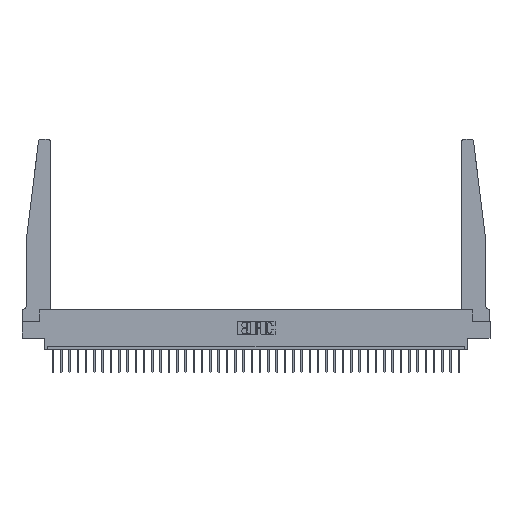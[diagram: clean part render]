
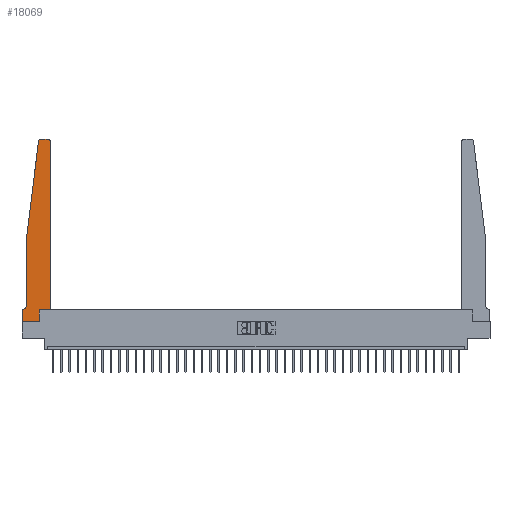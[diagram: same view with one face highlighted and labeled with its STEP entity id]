
A CAD part, top view. The second image highlights one B-rep face of the part: STEP entity #18069.
In plain terms, the highlighted planar face has unit normal (0, 0, 1).
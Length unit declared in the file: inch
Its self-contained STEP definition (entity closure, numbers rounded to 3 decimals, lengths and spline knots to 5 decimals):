
#10 = AXIS2_PLACEMENT_3D ( 'NONE', #720, #8918, #19592 ) ;
#615 = EDGE_CURVE ( 'NONE', #26898, #22682, #21179, .T. ) ;
#720 = CARTESIAN_POINT ( 'NONE',  ( 0.015, 0.2375, 0.37 ) ) ;
#728 = DIRECTION ( 'NONE',  ( 0., 0., 1. ) ) ;
#756 = CARTESIAN_POINT ( 'NONE',  ( 0.065, 1.25, 0.37 ) ) ;
#1066 = EDGE_CURVE ( 'NONE', #21076, #34703, #13447, .T. ) ;
#1390 = CARTESIAN_POINT ( 'NONE',  ( 0.065, 1.25, 0.37 ) ) ;
#3433 = CARTESIAN_POINT ( 'NONE',  ( 0.395, 2.72, 0.37 ) ) ;
#3521 = VECTOR ( 'NONE', #23719, 39.37008 ) ;
#3682 = ORIENTED_EDGE ( 'NONE', *, *, #18280, .T. ) ;
#3773 = LINE ( 'NONE', #25490, #32810 ) ;
#3813 = LINE ( 'NONE', #27204, #4213 ) ;
#3854 = CARTESIAN_POINT ( 'NONE',  ( 0.2605, 0.18, 0.37 ) ) ;
#4213 = VECTOR ( 'NONE', #9031, 39.37008 ) ;
#4278 = VECTOR ( 'NONE', #23794, 39.37008 ) ;
#5318 = FACE_OUTER_BOUND ( 'NONE', #15963, .T. ) ;
#5450 = CARTESIAN_POINT ( 'NONE',  ( 0.395, 2.75, 0.37 ) ) ;
#5536 = AXIS2_PLACEMENT_3D ( 'NONE', #22133, #27551, #32898 ) ;
#6871 = VERTEX_POINT ( 'NONE', #5450 ) ;
#6881 = CARTESIAN_POINT ( 'NONE',  ( 0., 0.1875, 0.37 ) ) ;
#7096 = EDGE_CURVE ( 'NONE', #6871, #26602, #25084, .T. ) ;
#7295 = VECTOR ( 'NONE', #30083, 39.37008 ) ;
#7425 = CARTESIAN_POINT ( 'NONE',  ( 0.25, 2.75, 0.37 ) ) ;
#7874 = EDGE_CURVE ( 'NONE', #22682, #6871, #25843, .T. ) ;
#8105 = EDGE_CURVE ( 'NONE', #16334, #30587, #10116, .T. ) ;
#8477 = DIRECTION ( 'NONE',  ( 1., 0., 0. ) ) ;
#8872 = ORIENTED_EDGE ( 'NONE', *, *, #16478, .T. ) ;
#8918 = DIRECTION ( 'NONE',  ( 0., 0., -1. ) ) ;
#9031 = DIRECTION ( 'NONE',  ( 1., 0., 0. ) ) ;
#9131 = EDGE_CURVE ( 'NONE', #26602, #26366, #9132, .T. ) ;
#9132 = CIRCLE ( 'NONE', #5536, 0.03 ) ;
#10116 = LINE ( 'NONE', #12217, #24058 ) ;
#10539 = CARTESIAN_POINT ( 'NONE',  ( 0.065, 0.2375, 0.37 ) ) ;
#11966 = DIRECTION ( 'NONE',  ( -0.122, -0.992, 0. ) ) ;
#12217 = CARTESIAN_POINT ( 'NONE',  ( 0.2605, 0.18, 0.37 ) ) ;
#12418 = EDGE_CURVE ( 'NONE', #34703, #12949, #14433, .T. ) ;
#12897 = CARTESIAN_POINT ( 'NONE',  ( 0.425, 0.18, 0.37 ) ) ;
#12949 = VERTEX_POINT ( 'NONE', #13727 ) ;
#13447 = CIRCLE ( 'NONE', #10, 0.05 ) ;
#13727 = CARTESIAN_POINT ( 'NONE',  ( 0., 0.1875, 0.37 ) ) ;
#14256 = CARTESIAN_POINT ( 'NONE',  ( 0., 0., 0.37 ) ) ;
#14433 = LINE ( 'NONE', #29742, #7295 ) ;
#15963 = EDGE_LOOP ( 'NONE', ( #25971, #26624, #28560, #3682, #24715, #16882, #20227, #16541, #18904, #8872, #28590, #29167 ) ) ;
#16064 = CARTESIAN_POINT ( 'NONE',  ( 0.425, 0.18, 0.37 ) ) ;
#16334 = VERTEX_POINT ( 'NONE', #25693 ) ;
#16478 = EDGE_CURVE ( 'NONE', #30587, #26898, #27355, .T. ) ;
#16541 = ORIENTED_EDGE ( 'NONE', *, *, #24718, .T. ) ;
#16688 = VERTEX_POINT ( 'NONE', #756 ) ;
#16882 = ORIENTED_EDGE ( 'NONE', *, *, #12418, .T. ) ;
#17820 = DIRECTION ( 'NONE',  ( 0., 1., 0. ) ) ;
#18069 = ADVANCED_FACE ( 'NONE', ( #5318 ), #22808, .T. ) ;
#18280 = EDGE_CURVE ( 'NONE', #16688, #21076, #22176, .T. ) ;
#18421 = VERTEX_POINT ( 'NONE', #14256 ) ;
#18584 = CARTESIAN_POINT ( 'NONE',  ( 0.015, 0.1875, 0.37 ) ) ;
#18609 = DIRECTION ( 'NONE',  ( 1., 0., 0. ) ) ;
#18716 = DIRECTION ( 'NONE',  ( 0., 0., 1. ) ) ;
#18904 = ORIENTED_EDGE ( 'NONE', *, *, #8105, .T. ) ;
#19592 = DIRECTION ( 'NONE',  ( -1., 0., 0. ) ) ;
#20227 = ORIENTED_EDGE ( 'NONE', *, *, #25146, .T. ) ;
#20305 = DIRECTION ( 'NONE',  ( 0., -1., 0. ) ) ;
#20562 = EDGE_CURVE ( 'NONE', #26366, #16688, #30845, .T. ) ;
#20798 = AXIS2_PLACEMENT_3D ( 'NONE', #3433, #728, #8477 ) ;
#21076 = VERTEX_POINT ( 'NONE', #10539 ) ;
#21179 = LINE ( 'NONE', #12897, #4278 ) ;
#22133 = CARTESIAN_POINT ( 'NONE',  ( 0.27653, 2.72, 0.37 ) ) ;
#22176 = LINE ( 'NONE', #1390, #32239 ) ;
#22188 = AXIS2_PLACEMENT_3D ( 'NONE', #6881, #18716, #18609 ) ;
#22682 = VERTEX_POINT ( 'NONE', #23199 ) ;
#22808 = PLANE ( 'NONE',  #22188 ) ;
#23199 = CARTESIAN_POINT ( 'NONE',  ( 0.425, 2.72, 0.37 ) ) ;
#23719 = DIRECTION ( 'NONE',  ( -1., 0., 0. ) ) ;
#23794 = DIRECTION ( 'NONE',  ( 0., 1., 0. ) ) ;
#24058 = VECTOR ( 'NONE', #17820, 39.37008 ) ;
#24235 = CARTESIAN_POINT ( 'NONE',  ( 0.24675, 2.72367, 0.37 ) ) ;
#24322 = CARTESIAN_POINT ( 'NONE',  ( 0.27653, 2.75, 0.37 ) ) ;
#24715 = ORIENTED_EDGE ( 'NONE', *, *, #1066, .T. ) ;
#24718 = EDGE_CURVE ( 'NONE', #18421, #16334, #3813, .T. ) ;
#25028 = DIRECTION ( 'NONE',  ( 0., -1., 0. ) ) ;
#25084 = LINE ( 'NONE', #7425, #3521 ) ;
#25146 = EDGE_CURVE ( 'NONE', #12949, #18421, #3773, .T. ) ;
#25490 = CARTESIAN_POINT ( 'NONE',  ( 0., 0., 0.37 ) ) ;
#25693 = CARTESIAN_POINT ( 'NONE',  ( 0.2605, 0., 0.37 ) ) ;
#25843 = CIRCLE ( 'NONE', #20798, 0.03 ) ;
#25971 = ORIENTED_EDGE ( 'NONE', *, *, #7096, .T. ) ;
#26366 = VERTEX_POINT ( 'NONE', #24235 ) ;
#26602 = VERTEX_POINT ( 'NONE', #24322 ) ;
#26619 = CARTESIAN_POINT ( 'NONE',  ( 0.425, 0.18, 0.37 ) ) ;
#26624 = ORIENTED_EDGE ( 'NONE', *, *, #9131, .T. ) ;
#26898 = VERTEX_POINT ( 'NONE', #16064 ) ;
#27204 = CARTESIAN_POINT ( 'NONE',  ( 0., 0., 0.37 ) ) ;
#27355 = LINE ( 'NONE', #26619, #29046 ) ;
#27551 = DIRECTION ( 'NONE',  ( 0., 0., 1. ) ) ;
#28560 = ORIENTED_EDGE ( 'NONE', *, *, #20562, .T. ) ;
#28590 = ORIENTED_EDGE ( 'NONE', *, *, #615, .T. ) ;
#29046 = VECTOR ( 'NONE', #34427, 39.37008 ) ;
#29167 = ORIENTED_EDGE ( 'NONE', *, *, #7874, .T. ) ;
#29188 = VECTOR ( 'NONE', #11966, 39.37008 ) ;
#29742 = CARTESIAN_POINT ( 'NONE',  ( 0.065, 0.1875, 0.37 ) ) ;
#30083 = DIRECTION ( 'NONE',  ( -1., 0., 0. ) ) ;
#30587 = VERTEX_POINT ( 'NONE', #3854 ) ;
#30845 = LINE ( 'NONE', #33503, #29188 ) ;
#32239 = VECTOR ( 'NONE', #20305, 39.37008 ) ;
#32810 = VECTOR ( 'NONE', #25028, 39.37008 ) ;
#32898 = DIRECTION ( 'NONE',  ( 1., 0., 0. ) ) ;
#33503 = CARTESIAN_POINT ( 'NONE',  ( 0.065, 1.25, 0.37 ) ) ;
#34427 = DIRECTION ( 'NONE',  ( 1., 0., 0. ) ) ;
#34703 = VERTEX_POINT ( 'NONE', #18584 ) ;
